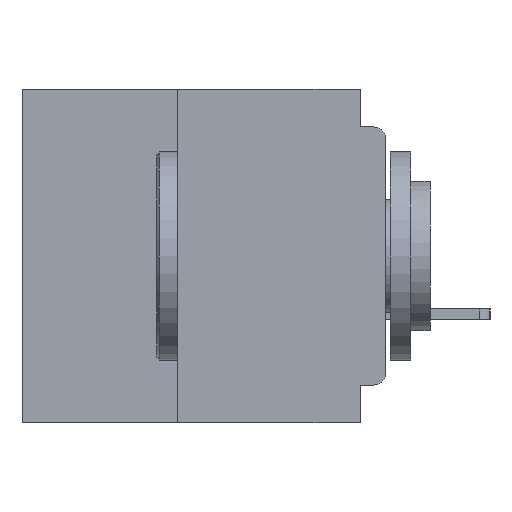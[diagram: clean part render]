
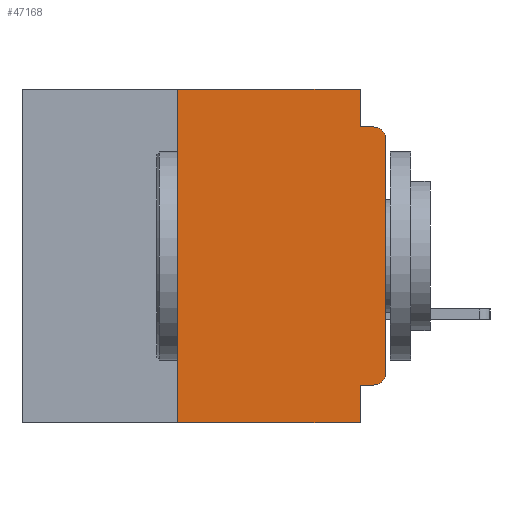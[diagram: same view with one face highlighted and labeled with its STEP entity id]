
A CAD part, left-side view. The second image highlights one B-rep face of the part: STEP entity #47168.
In plain terms, the highlighted planar face has unit normal (-1, 0, 0).
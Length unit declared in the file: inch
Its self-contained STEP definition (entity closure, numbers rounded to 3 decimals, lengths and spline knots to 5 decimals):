
#143 = LINE ( 'NONE', #45292, #9767 ) ;
#533 = LINE ( 'NONE', #34225, #42495 ) ;
#765 = AXIS2_PLACEMENT_3D ( 'NONE', #32216, #7936, #36307 ) ;
#865 = VERTEX_POINT ( 'NONE', #18647 ) ;
#2037 = VECTOR ( 'NONE', #30207, 39.37008 ) ;
#2595 = DIRECTION ( 'NONE',  ( -1., 0., 0. ) ) ;
#3196 = DIRECTION ( 'NONE',  ( 0., 0., 1. ) ) ;
#5695 = EDGE_CURVE ( 'NONE', #26651, #34098, #46044, .T. ) ;
#5700 = PLANE ( 'NONE',  #10402 ) ;
#5926 = DIRECTION ( 'NONE',  ( 0., -1., 0. ) ) ;
#6890 = ORIENTED_EDGE ( 'NONE', *, *, #14187, .T. ) ;
#7339 = ORIENTED_EDGE ( 'NONE', *, *, #29394, .F. ) ;
#7589 = EDGE_CURVE ( 'NONE', #12518, #36737, #48974, .T. ) ;
#7607 = VERTEX_POINT ( 'NONE', #31399 ) ;
#7936 = DIRECTION ( 'NONE',  ( -1., 0., 0. ) ) ;
#8434 = ORIENTED_EDGE ( 'NONE', *, *, #7589, .F. ) ;
#8916 = EDGE_CURVE ( 'NONE', #42159, #7607, #40086, .T. ) ;
#8956 = DIRECTION ( 'NONE',  ( 0., 1., 0. ) ) ;
#9405 = ORIENTED_EDGE ( 'NONE', *, *, #29558, .T. ) ;
#9767 = VECTOR ( 'NONE', #8956, 39.37008 ) ;
#9834 = DIRECTION ( 'NONE',  ( 0., 0., -1. ) ) ;
#10402 = AXIS2_PLACEMENT_3D ( 'NONE', #42084, #34084, #9834 ) ;
#12207 = ORIENTED_EDGE ( 'NONE', *, *, #40435, .F. ) ;
#12518 = VERTEX_POINT ( 'NONE', #24429 ) ;
#12781 = VECTOR ( 'NONE', #27144, 39.37008 ) ;
#14000 = AXIS2_PLACEMENT_3D ( 'NONE', #26976, #2595, #31043 ) ;
#14187 = EDGE_CURVE ( 'NONE', #22202, #34098, #48588, .T. ) ;
#15192 = DIRECTION ( 'NONE',  ( 0., 0., -1. ) ) ;
#16490 = LINE ( 'NONE', #32821, #36734 ) ;
#17499 = CARTESIAN_POINT ( 'NONE',  ( 0., 0.015, -0.045 ) ) ;
#18647 = CARTESIAN_POINT ( 'NONE',  ( 0., 0.25, -0.4 ) ) ;
#19077 = CARTESIAN_POINT ( 'NONE',  ( 0., 0.031, -0.4 ) ) ;
#19170 = EDGE_CURVE ( 'NONE', #865, #36723, #16490, .T. ) ;
#22148 = CARTESIAN_POINT ( 'NONE',  ( 0., 0., -0.045 ) ) ;
#22202 = VERTEX_POINT ( 'NONE', #26679 ) ;
#22712 = ORIENTED_EDGE ( 'NONE', *, *, #19170, .F. ) ;
#23133 = CARTESIAN_POINT ( 'NONE',  ( 0., 0.031, -0.4 ) ) ;
#23734 = LINE ( 'NONE', #34261, #2037 ) ;
#24137 = EDGE_CURVE ( 'NONE', #7607, #22202, #51131, .T. ) ;
#24429 = CARTESIAN_POINT ( 'NONE',  ( 0., 0.031, -0.355 ) ) ;
#24744 = ORIENTED_EDGE ( 'NONE', *, *, #24137, .T. ) ;
#26625 = CARTESIAN_POINT ( 'NONE',  ( 0., 0.015, -0.355 ) ) ;
#26651 = VERTEX_POINT ( 'NONE', #35295 ) ;
#26679 = CARTESIAN_POINT ( 'NONE',  ( 0., 0., -0.06 ) ) ;
#26976 = CARTESIAN_POINT ( 'NONE',  ( 0., 0.015, -0.34 ) ) ;
#27035 = VERTEX_POINT ( 'NONE', #49796 ) ;
#27144 = DIRECTION ( 'NONE',  ( 0., -1., 0. ) ) ;
#27410 = ORIENTED_EDGE ( 'NONE', *, *, #42253, .F. ) ;
#29148 = FACE_OUTER_BOUND ( 'NONE', #34486, .T. ) ;
#29394 = EDGE_CURVE ( 'NONE', #42159, #12518, #143, .T. ) ;
#29558 = EDGE_CURVE ( 'NONE', #865, #36737, #23734, .T. ) ;
#29607 = VECTOR ( 'NONE', #3196, 39.37008 ) ;
#30207 = DIRECTION ( 'NONE',  ( 0., -1., 0. ) ) ;
#31043 = DIRECTION ( 'NONE',  ( 0., 0., -1. ) ) ;
#31399 = CARTESIAN_POINT ( 'NONE',  ( 0., 0., -0.34 ) ) ;
#32216 = CARTESIAN_POINT ( 'NONE',  ( 0., 0.015, -0.06 ) ) ;
#32763 = ORIENTED_EDGE ( 'NONE', *, *, #5695, .F. ) ;
#32821 = CARTESIAN_POINT ( 'NONE',  ( 0., 0.25, -0.4 ) ) ;
#34048 = DIRECTION ( 'NONE',  ( 0., 0., -1. ) ) ;
#34084 = DIRECTION ( 'NONE',  ( 1., 0., 0. ) ) ;
#34098 = VERTEX_POINT ( 'NONE', #17499 ) ;
#34225 = CARTESIAN_POINT ( 'NONE',  ( 0., 0.031, 0. ) ) ;
#34261 = CARTESIAN_POINT ( 'NONE',  ( 0., 0.437, -0.4 ) ) ;
#34486 = EDGE_LOOP ( 'NONE', ( #24744, #6890, #32763, #12207, #27410, #22712, #9405, #8434, #7339, #40225 ) ) ;
#35230 = VECTOR ( 'NONE', #5926, 39.37008 ) ;
#35295 = CARTESIAN_POINT ( 'NONE',  ( 0., 0.031, -0.045 ) ) ;
#36307 = DIRECTION ( 'NONE',  ( 0., 0., -1. ) ) ;
#36723 = VERTEX_POINT ( 'NONE', #51213 ) ;
#36734 = VECTOR ( 'NONE', #36939, 39.37008 ) ;
#36737 = VERTEX_POINT ( 'NONE', #19077 ) ;
#36939 = DIRECTION ( 'NONE',  ( 0., 0., 1. ) ) ;
#38225 = VECTOR ( 'NONE', #15192, 39.37008 ) ;
#40086 = CIRCLE ( 'NONE', #14000, 0.015 ) ;
#40225 = ORIENTED_EDGE ( 'NONE', *, *, #8916, .T. ) ;
#40435 = EDGE_CURVE ( 'NONE', #27035, #26651, #533, .T. ) ;
#42084 = CARTESIAN_POINT ( 'NONE',  ( 0., 0.437, 0. ) ) ;
#42159 = VERTEX_POINT ( 'NONE', #26625 ) ;
#42253 = EDGE_CURVE ( 'NONE', #36723, #27035, #46364, .T. ) ;
#42495 = VECTOR ( 'NONE', #34048, 39.37008 ) ;
#45292 = CARTESIAN_POINT ( 'NONE',  ( 0., 0., -0.355 ) ) ;
#46044 = LINE ( 'NONE', #22148, #35230 ) ;
#46364 = LINE ( 'NONE', #47368, #12781 ) ;
#47168 = ADVANCED_FACE ( 'NONE', ( #29148 ), #5700, .F. ) ;
#47368 = CARTESIAN_POINT ( 'NONE',  ( 0., 0.437, 0. ) ) ;
#47771 = CARTESIAN_POINT ( 'NONE',  ( 0., 0., 0. ) ) ;
#48588 = CIRCLE ( 'NONE', #765, 0.015 ) ;
#48974 = LINE ( 'NONE', #23133, #38225 ) ;
#49796 = CARTESIAN_POINT ( 'NONE',  ( 0., 0.031, 0. ) ) ;
#51131 = LINE ( 'NONE', #47771, #29607 ) ;
#51213 = CARTESIAN_POINT ( 'NONE',  ( 0., 0.25, 0. ) ) ;
